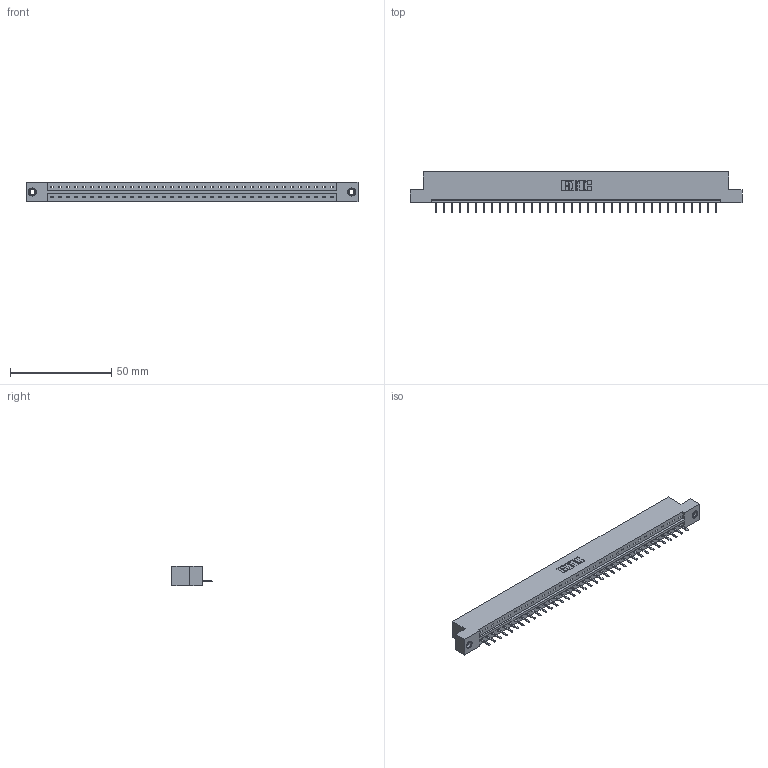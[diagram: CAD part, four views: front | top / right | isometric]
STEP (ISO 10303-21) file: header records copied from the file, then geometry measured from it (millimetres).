
FILE_DESCRIPTION (( 'STEP AP203' ), '1' );
FILE_NAME ('333-036-520-107.STEP', '2018-08-03T00:14:31', ( '' ), ( '' ), 'SwSTEP 2.0', 'SolidWorks 2016', '' );
FILE_SCHEMA (( 'CONFIG_CONTROL_DESIGN' ));
Length unit declared in the file: inch
Products named in the file (4): 345-292-001_345-293-120; 345-250-001_345-250-005-103; 333-036-520-107; 333 Part_Flush - .156 Dia - TI
Assembly tree (39 placements, depth 2):
  333-036-520-107
    333 Part_Flush - .156 Dia - TI
    345-292-001_345-293-120  x36
    345-250-001_345-250-005-103  x2
Bounding box: 164.19 x 20.02 x 9.4 mm (x, y, z)
Volume: 16353 mm3; surface area: 17328.7 mm2
Topology: 39 solids, 39 shells, 2406 faces, 7071 edges, 4610 vertices
Faces by surface type: plane 1686, cylinder 704, cone 12, torus 4
Entity records: 24084 total; most frequent: CARTESIAN_POINT 4149, ORIENTED_EDGE 4102, DIRECTION 3533, EDGE_CURVE 2051, LINE 1899, VECTOR 1899, VERTEX_POINT 1360, AXIS2_PLACEMENT_3D 817
